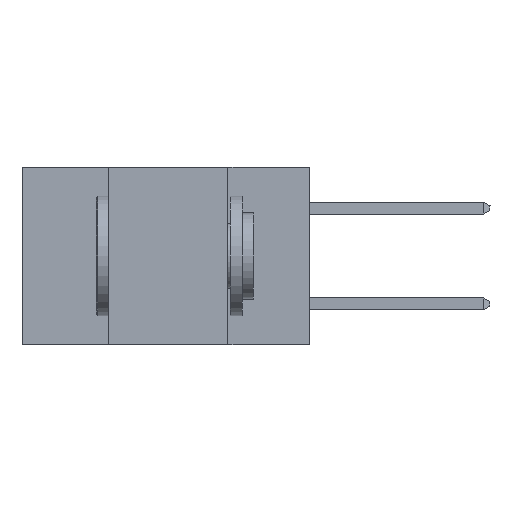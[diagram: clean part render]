
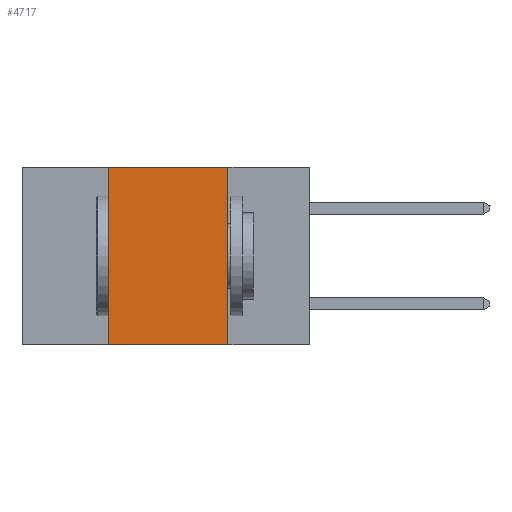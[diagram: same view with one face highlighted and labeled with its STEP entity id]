
A CAD part, left-side view. The second image highlights one B-rep face of the part: STEP entity #4717.
In plain terms, the highlighted planar face has unit normal (-1, 0, 0).
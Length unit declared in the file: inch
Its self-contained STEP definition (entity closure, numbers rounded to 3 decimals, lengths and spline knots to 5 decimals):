
#33 = VERTEX_POINT ( 'NONE', #12063 ) ;
#1006 = VECTOR ( 'NONE', #2357, 39.37008 ) ;
#1910 = DIRECTION ( 'NONE',  ( 0., 0., 1. ) ) ;
#2357 = DIRECTION ( 'NONE',  ( 0., -1., 0. ) ) ;
#3275 = VECTOR ( 'NONE', #1910, 39.37008 ) ;
#4083 = CARTESIAN_POINT ( 'NONE',  ( 0., 0.42, 0. ) ) ;
#4281 = LINE ( 'NONE', #9693, #1006 ) ;
#4552 = ORIENTED_EDGE ( 'NONE', *, *, #11311, .F. ) ;
#4665 = VECTOR ( 'NONE', #6041, 39.37008 ) ;
#4717 = ADVANCED_FACE ( 'NONE', ( #6976 ), #13376, .F. ) ;
#4937 = ORIENTED_EDGE ( 'NONE', *, *, #13873, .F. ) ;
#5043 = ORIENTED_EDGE ( 'NONE', *, *, #9213, .T. ) ;
#5045 = LINE ( 'NONE', #7211, #4665 ) ;
#5181 = VERTEX_POINT ( 'NONE', #12742 ) ;
#5334 = EDGE_LOOP ( 'NONE', ( #7735, #4937, #4552, #5043 ) ) ;
#5338 = VERTEX_POINT ( 'NONE', #7191 ) ;
#5660 = AXIS2_PLACEMENT_3D ( 'NONE', #13281, #11586, #11569 ) ;
#5774 = VERTEX_POINT ( 'NONE', #4083 ) ;
#6041 = DIRECTION ( 'NONE',  ( 0., -1., 0. ) ) ;
#6734 = VECTOR ( 'NONE', #7963, 39.37008 ) ;
#6976 = FACE_OUTER_BOUND ( 'NONE', #5334, .T. ) ;
#7191 = CARTESIAN_POINT ( 'NONE',  ( 0., 0.17, -0.37 ) ) ;
#7211 = CARTESIAN_POINT ( 'NONE',  ( 0., 0.6, 0. ) ) ;
#7735 = ORIENTED_EDGE ( 'NONE', *, *, #12620, .F. ) ;
#7963 = DIRECTION ( 'NONE',  ( 0., 0., -1. ) ) ;
#9175 = CARTESIAN_POINT ( 'NONE',  ( 0., 0.17, 0. ) ) ;
#9213 = EDGE_CURVE ( 'NONE', #5181, #5338, #4281, .T. ) ;
#9693 = CARTESIAN_POINT ( 'NONE',  ( 0., 0.6, -0.37 ) ) ;
#10680 = LINE ( 'NONE', #9175, #6734 ) ;
#11311 = EDGE_CURVE ( 'NONE', #5181, #5774, #12798, .T. ) ;
#11569 = DIRECTION ( 'NONE',  ( 0., 0., -1. ) ) ;
#11586 = DIRECTION ( 'NONE',  ( 1., 0., 0. ) ) ;
#12063 = CARTESIAN_POINT ( 'NONE',  ( 0., 0.17, 0. ) ) ;
#12620 = EDGE_CURVE ( 'NONE', #33, #5338, #10680, .T. ) ;
#12742 = CARTESIAN_POINT ( 'NONE',  ( 0., 0.42, -0.37 ) ) ;
#12766 = CARTESIAN_POINT ( 'NONE',  ( 0., 0.42, 0. ) ) ;
#12798 = LINE ( 'NONE', #12766, #3275 ) ;
#13281 = CARTESIAN_POINT ( 'NONE',  ( 0., 0.6, 0. ) ) ;
#13376 = PLANE ( 'NONE',  #5660 ) ;
#13873 = EDGE_CURVE ( 'NONE', #5774, #33, #5045, .T. ) ;
